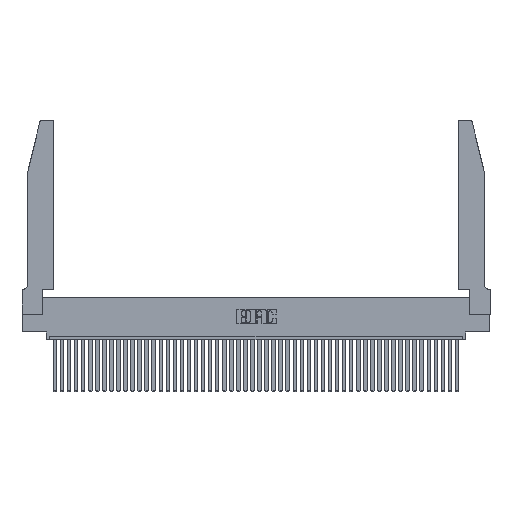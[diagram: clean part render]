
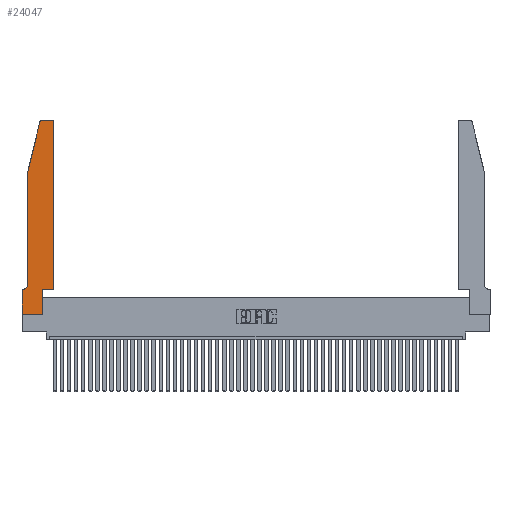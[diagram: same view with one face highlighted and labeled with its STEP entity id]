
A CAD part, top view. The second image highlights one B-rep face of the part: STEP entity #24047.
In plain terms, the highlighted planar face has unit normal (0, 0, 1).
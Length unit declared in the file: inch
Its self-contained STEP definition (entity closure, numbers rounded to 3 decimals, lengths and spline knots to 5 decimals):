
#16 = ORIENTED_EDGE ( 'NONE', *, *, #44273, .T. ) ;
#482 = DIRECTION ( 'NONE',  ( -1., 0., 0. ) ) ;
#495 = CARTESIAN_POINT ( 'NONE',  ( 0.2865, 0.35, 0.37 ) ) ;
#1130 = CARTESIAN_POINT ( 'NONE',  ( 0., 0., 0.37 ) ) ;
#2072 = VERTEX_POINT ( 'NONE', #2132 ) ;
#2132 = CARTESIAN_POINT ( 'NONE',  ( 0.0755, 2., 0.37 ) ) ;
#3407 = VECTOR ( 'NONE', #35717, 39.37008 ) ;
#3555 = AXIS2_PLACEMENT_3D ( 'NONE', #19096, #28001, #12281 ) ;
#3765 = VECTOR ( 'NONE', #15157, 39.37008 ) ;
#4340 = VECTOR ( 'NONE', #482, 39.37008 ) ;
#4503 = EDGE_CURVE ( 'NONE', #13290, #14726, #25839, .T. ) ;
#6764 = CARTESIAN_POINT ( 'NONE',  ( 0.2605, 2.75, 0.37 ) ) ;
#7735 = CARTESIAN_POINT ( 'NONE',  ( 0.0755, 2., 0.37 ) ) ;
#7740 = VECTOR ( 'NONE', #31691, 39.37008 ) ;
#8107 = PLANE ( 'NONE',  #3555 ) ;
#8627 = CARTESIAN_POINT ( 'NONE',  ( 0.4205, 2.72, 0.37 ) ) ;
#9596 = EDGE_CURVE ( 'NONE', #36706, #30475, #19141, .T. ) ;
#9793 = VECTOR ( 'NONE', #23787, 39.37008 ) ;
#10252 = CARTESIAN_POINT ( 'NONE',  ( 0.2865, 0.35, 0.37 ) ) ;
#10348 = EDGE_CURVE ( 'NONE', #33990, #2072, #14084, .T. ) ;
#11074 = VECTOR ( 'NONE', #39330, 39.37008 ) ;
#11456 = VERTEX_POINT ( 'NONE', #43173 ) ;
#12281 = DIRECTION ( 'NONE',  ( 1., 0., 0. ) ) ;
#12404 = CARTESIAN_POINT ( 'NONE',  ( 0.0755, 0.42, 0.37 ) ) ;
#13026 = CARTESIAN_POINT ( 'NONE',  ( 0.4505, 0.35, 0.37 ) ) ;
#13290 = VERTEX_POINT ( 'NONE', #30732 ) ;
#13918 = CARTESIAN_POINT ( 'NONE',  ( 0., 0., 0.37 ) ) ;
#13976 = CARTESIAN_POINT ( 'NONE',  ( 0.4505, 0.35, 0.37 ) ) ;
#13985 = VECTOR ( 'NONE', #41523, 39.37008 ) ;
#14007 = LINE ( 'NONE', #13918, #3407 ) ;
#14084 = LINE ( 'NONE', #30295, #17429 ) ;
#14388 = ORIENTED_EDGE ( 'NONE', *, *, #35383, .T. ) ;
#14726 = VERTEX_POINT ( 'NONE', #40378 ) ;
#15157 = DIRECTION ( 'NONE',  ( 0., -1., 0. ) ) ;
#15433 = DIRECTION ( 'NONE',  ( 1., 0., 0. ) ) ;
#15663 = VERTEX_POINT ( 'NONE', #30382 ) ;
#16471 = AXIS2_PLACEMENT_3D ( 'NONE', #8627, #33512, #44764 ) ;
#17116 = AXIS2_PLACEMENT_3D ( 'NONE', #29739, #40534, #15433 ) ;
#17429 = VECTOR ( 'NONE', #26183, 39.37008 ) ;
#17966 = ORIENTED_EDGE ( 'NONE', *, *, #44883, .T. ) ;
#19096 = CARTESIAN_POINT ( 'NONE',  ( 0., 0.35, 0.37 ) ) ;
#19141 = LINE ( 'NONE', #45218, #9793 ) ;
#19612 = AXIS2_PLACEMENT_3D ( 'NONE', #34770, #38337, #23483 ) ;
#19717 = ORIENTED_EDGE ( 'NONE', *, *, #19999, .T. ) ;
#19971 = LINE ( 'NONE', #10252, #7740 ) ;
#19999 = EDGE_CURVE ( 'NONE', #2072, #20860, #35011, .T. ) ;
#20285 = EDGE_CURVE ( 'NONE', #43247, #13290, #41279, .T. ) ;
#20510 = CARTESIAN_POINT ( 'NONE',  ( 0.25487, 2.72718, 0.37 ) ) ;
#20860 = VERTEX_POINT ( 'NONE', #12404 ) ;
#21072 = EDGE_CURVE ( 'NONE', #30475, #39574, #19971, .T. ) ;
#23191 = CIRCLE ( 'NONE', #17116, 0.03 ) ;
#23483 = DIRECTION ( 'NONE',  ( -1., 0., 0. ) ) ;
#23784 = ORIENTED_EDGE ( 'NONE', *, *, #24499, .T. ) ;
#23787 = DIRECTION ( 'NONE',  ( 1., 0., 0. ) ) ;
#24047 = ADVANCED_FACE ( 'NONE', ( #40314 ), #8107, .T. ) ;
#24499 = EDGE_CURVE ( 'NONE', #14726, #15663, #28546, .T. ) ;
#25839 = CIRCLE ( 'NONE', #16471, 0.03 ) ;
#26172 = ORIENTED_EDGE ( 'NONE', *, *, #21072, .T. ) ;
#26183 = DIRECTION ( 'NONE',  ( -0.239, -0.971, 0. ) ) ;
#26207 = ORIENTED_EDGE ( 'NONE', *, *, #36636, .T. ) ;
#28001 = DIRECTION ( 'NONE',  ( 0., 0., 1. ) ) ;
#28546 = LINE ( 'NONE', #6764, #44789 ) ;
#29739 = CARTESIAN_POINT ( 'NONE',  ( 0.284, 2.72, 0.37 ) ) ;
#29897 = CARTESIAN_POINT ( 'NONE',  ( 0., 0.35, 0.37 ) ) ;
#30295 = CARTESIAN_POINT ( 'NONE',  ( 0.0755, 2., 0.37 ) ) ;
#30382 = CARTESIAN_POINT ( 'NONE',  ( 0.284, 2.75, 0.37 ) ) ;
#30475 = VERTEX_POINT ( 'NONE', #33723 ) ;
#30732 = CARTESIAN_POINT ( 'NONE',  ( 0.4505, 2.72, 0.37 ) ) ;
#31017 = EDGE_LOOP ( 'NONE', ( #23784, #17966, #33042, #19717, #38198, #26207, #14388, #39057, #26172, #16, #31217, #37546 ) ) ;
#31217 = ORIENTED_EDGE ( 'NONE', *, *, #20285, .T. ) ;
#31691 = DIRECTION ( 'NONE',  ( 0., 1., 0. ) ) ;
#33042 = ORIENTED_EDGE ( 'NONE', *, *, #10348, .T. ) ;
#33512 = DIRECTION ( 'NONE',  ( 0., 0., 1. ) ) ;
#33723 = CARTESIAN_POINT ( 'NONE',  ( 0.2865, 0., 0.37 ) ) ;
#33962 = EDGE_CURVE ( 'NONE', #20860, #11456, #38685, .T. ) ;
#33990 = VERTEX_POINT ( 'NONE', #20510 ) ;
#34770 = CARTESIAN_POINT ( 'NONE',  ( 0.0055, 0.42, 0.37 ) ) ;
#35011 = LINE ( 'NONE', #7735, #3765 ) ;
#35383 = EDGE_CURVE ( 'NONE', #37419, #36706, #14007, .T. ) ;
#35717 = DIRECTION ( 'NONE',  ( 0., -1., 0. ) ) ;
#35847 = DIRECTION ( 'NONE',  ( -1., 0., 0. ) ) ;
#36110 = LINE ( 'NONE', #13976, #11074 ) ;
#36636 = EDGE_CURVE ( 'NONE', #11456, #37419, #42331, .T. ) ;
#36706 = VERTEX_POINT ( 'NONE', #1130 ) ;
#37419 = VERTEX_POINT ( 'NONE', #29897 ) ;
#37546 = ORIENTED_EDGE ( 'NONE', *, *, #4503, .T. ) ;
#38198 = ORIENTED_EDGE ( 'NONE', *, *, #33962, .T. ) ;
#38337 = DIRECTION ( 'NONE',  ( 0., 0., -1. ) ) ;
#38685 = CIRCLE ( 'NONE', #19612, 0.07 ) ;
#39057 = ORIENTED_EDGE ( 'NONE', *, *, #9596, .T. ) ;
#39330 = DIRECTION ( 'NONE',  ( 1., 0., 0. ) ) ;
#39574 = VERTEX_POINT ( 'NONE', #495 ) ;
#40314 = FACE_OUTER_BOUND ( 'NONE', #31017, .T. ) ;
#40378 = CARTESIAN_POINT ( 'NONE',  ( 0.4205, 2.75, 0.37 ) ) ;
#40534 = DIRECTION ( 'NONE',  ( 0., 0., 1. ) ) ;
#41279 = LINE ( 'NONE', #13026, #13985 ) ;
#41523 = DIRECTION ( 'NONE',  ( 0., 1., 0. ) ) ;
#41624 = CARTESIAN_POINT ( 'NONE',  ( 0.0755, 0.35, 0.37 ) ) ;
#42331 = LINE ( 'NONE', #41624, #4340 ) ;
#43173 = CARTESIAN_POINT ( 'NONE',  ( 0.0055, 0.35, 0.37 ) ) ;
#43247 = VERTEX_POINT ( 'NONE', #44252 ) ;
#44252 = CARTESIAN_POINT ( 'NONE',  ( 0.4505, 0.35, 0.37 ) ) ;
#44273 = EDGE_CURVE ( 'NONE', #39574, #43247, #36110, .T. ) ;
#44764 = DIRECTION ( 'NONE',  ( 1., 0., 0. ) ) ;
#44789 = VECTOR ( 'NONE', #35847, 39.37008 ) ;
#44883 = EDGE_CURVE ( 'NONE', #15663, #33990, #23191, .T. ) ;
#45218 = CARTESIAN_POINT ( 'NONE',  ( 0., 0., 0.37 ) ) ;
